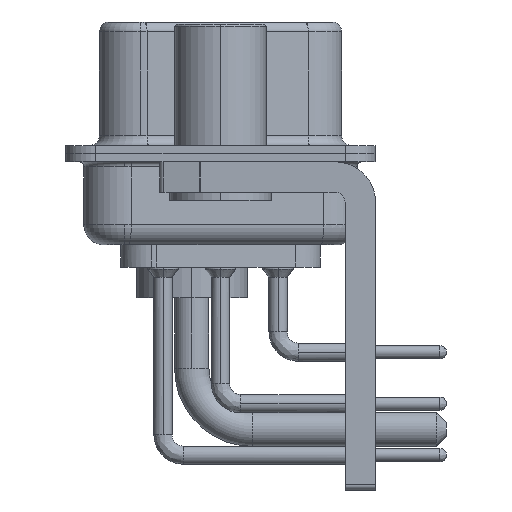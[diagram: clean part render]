
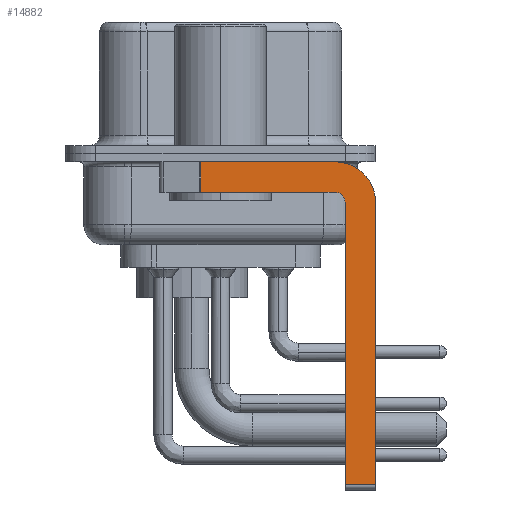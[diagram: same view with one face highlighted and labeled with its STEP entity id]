
A CAD part, left-side view. The second image highlights one B-rep face of the part: STEP entity #14882.
In plain terms, the highlighted planar face has unit normal (-1, 0, 0).
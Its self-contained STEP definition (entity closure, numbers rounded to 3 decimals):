
#856 = DIRECTION ( 'NONE',  ( 0., 0., 1. ) ) ;
#2683 = CARTESIAN_POINT ( 'NONE',  ( -2.9, -5.65, -1.9 ) ) ;
#3170 = CARTESIAN_POINT ( 'NONE',  ( -2.9, -5.65, -16.35 ) ) ;
#4064 = VERTEX_POINT ( 'NONE', #15832 ) ;
#4193 = ORIENTED_EDGE ( 'NONE', *, *, #4980, .F. ) ;
#4289 = DIRECTION ( 'NONE',  ( 0., 0., -1. ) ) ;
#4336 = ORIENTED_EDGE ( 'NONE', *, *, #36828, .F. ) ;
#4679 = CARTESIAN_POINT ( 'NONE',  ( -2.9, -5.65, -2.4 ) ) ;
#4980 = EDGE_CURVE ( 'NONE', #4064, #15837, #27712, .T. ) ;
#5061 = DIRECTION ( 'NONE',  ( 0., 0., -1. ) ) ;
#6954 = EDGE_LOOP ( 'NONE', ( #4336, #30407, #34173, #9343, #15184, #26430, #28170, #4193 ) ) ;
#7166 = VERTEX_POINT ( 'NONE', #35338 ) ;
#7677 = CARTESIAN_POINT ( 'NONE',  ( -2.9, -5.65, -1.9 ) ) ;
#8299 = VERTEX_POINT ( 'NONE', #32173 ) ;
#8831 = VECTOR ( 'NONE', #9460, 1000. ) ;
#9119 = CARTESIAN_POINT ( 'NONE',  ( -2.9, 0.978, -1.9 ) ) ;
#9193 = VECTOR ( 'NONE', #5061, 1000. ) ;
#9343 = ORIENTED_EDGE ( 'NONE', *, *, #24892, .F. ) ;
#9460 = DIRECTION ( 'NONE',  ( 0., -1., 0. ) ) ;
#9918 = VECTOR ( 'NONE', #20905, 1000. ) ;
#10504 = DIRECTION ( 'NONE',  ( 0., 0., -1. ) ) ;
#10552 = DIRECTION ( 'NONE',  ( 1., 0., 0. ) ) ;
#10808 = CIRCLE ( 'NONE', #14056, 0.5 ) ;
#11308 = VECTOR ( 'NONE', #10504, 1000. ) ;
#13034 = CARTESIAN_POINT ( 'NONE',  ( -2.9, -5.65, -2.4 ) ) ;
#13354 = CARTESIAN_POINT ( 'NONE',  ( -2.9, 3., -0.4 ) ) ;
#13552 = LINE ( 'NONE', #25862, #11308 ) ;
#13935 = EDGE_CURVE ( 'NONE', #7166, #36675, #13552, .T. ) ;
#14056 = AXIS2_PLACEMENT_3D ( 'NONE', #13034, #19266, #856 ) ;
#14796 = VECTOR ( 'NONE', #25679, 1000. ) ;
#14882 = ADVANCED_FACE ( 'NONE', ( #31954 ), #38957, .F. ) ;
#15184 = ORIENTED_EDGE ( 'NONE', *, *, #31485, .F. ) ;
#15832 = CARTESIAN_POINT ( 'NONE',  ( -2.9, -5.65, -0.4 ) ) ;
#15837 = VERTEX_POINT ( 'NONE', #25497 ) ;
#18304 = VERTEX_POINT ( 'NONE', #18493 ) ;
#18493 = CARTESIAN_POINT ( 'NONE',  ( -2.9, -7.65, -16.35 ) ) ;
#19056 = VECTOR ( 'NONE', #25533, 1000. ) ;
#19202 = DIRECTION ( 'NONE',  ( 1., 0., 0. ) ) ;
#19266 = DIRECTION ( 'NONE',  ( -1., 0., 0. ) ) ;
#20905 = DIRECTION ( 'NONE',  ( 0., 1., 0. ) ) ;
#21751 = VERTEX_POINT ( 'NONE', #35544 ) ;
#22433 = EDGE_CURVE ( 'NONE', #8299, #18304, #34670, .T. ) ;
#24892 = EDGE_CURVE ( 'NONE', #21751, #35854, #10808, .T. ) ;
#25096 = DIRECTION ( 'NONE',  ( 0., 0., -1. ) ) ;
#25497 = CARTESIAN_POINT ( 'NONE',  ( -2.9, -7.65, -2.4 ) ) ;
#25533 = DIRECTION ( 'NONE',  ( 0., 0., 1. ) ) ;
#25679 = DIRECTION ( 'NONE',  ( 0., -1., 0. ) ) ;
#25862 = CARTESIAN_POINT ( 'NONE',  ( -2.9, 0.978, -1.9 ) ) ;
#26430 = ORIENTED_EDGE ( 'NONE', *, *, #22433, .T. ) ;
#27712 = CIRCLE ( 'NONE', #37381, 2. ) ;
#28170 = ORIENTED_EDGE ( 'NONE', *, *, #28637, .F. ) ;
#28637 = EDGE_CURVE ( 'NONE', #15837, #18304, #30325, .T. ) ;
#30012 = EDGE_CURVE ( 'NONE', #35854, #36675, #30182, .T. ) ;
#30182 = LINE ( 'NONE', #2683, #9918 ) ;
#30325 = LINE ( 'NONE', #38235, #9193 ) ;
#30407 = ORIENTED_EDGE ( 'NONE', *, *, #13935, .T. ) ;
#31361 = LINE ( 'NONE', #34967, #19056 ) ;
#31485 = EDGE_CURVE ( 'NONE', #8299, #21751, #31361, .T. ) ;
#31954 = FACE_OUTER_BOUND ( 'NONE', #6954, .T. ) ;
#32173 = CARTESIAN_POINT ( 'NONE',  ( -2.9, -6.15, -16.35 ) ) ;
#32315 = LINE ( 'NONE', #13354, #14796 ) ;
#34173 = ORIENTED_EDGE ( 'NONE', *, *, #30012, .F. ) ;
#34670 = LINE ( 'NONE', #3170, #8831 ) ;
#34921 = CARTESIAN_POINT ( 'NONE',  ( -2.9, -5.65, -2.4 ) ) ;
#34967 = CARTESIAN_POINT ( 'NONE',  ( -2.9, -6.15, -16.6 ) ) ;
#35338 = CARTESIAN_POINT ( 'NONE',  ( -2.9, 0.978, -0.4 ) ) ;
#35544 = CARTESIAN_POINT ( 'NONE',  ( -2.9, -6.15, -2.4 ) ) ;
#35854 = VERTEX_POINT ( 'NONE', #7677 ) ;
#36675 = VERTEX_POINT ( 'NONE', #9119 ) ;
#36770 = AXIS2_PLACEMENT_3D ( 'NONE', #4679, #10552, #4289 ) ;
#36828 = EDGE_CURVE ( 'NONE', #7166, #4064, #32315, .T. ) ;
#37381 = AXIS2_PLACEMENT_3D ( 'NONE', #34921, #19202, #25096 ) ;
#38235 = CARTESIAN_POINT ( 'NONE',  ( -2.9, -7.65, -2.4 ) ) ;
#38957 = PLANE ( 'NONE',  #36770 ) ;
